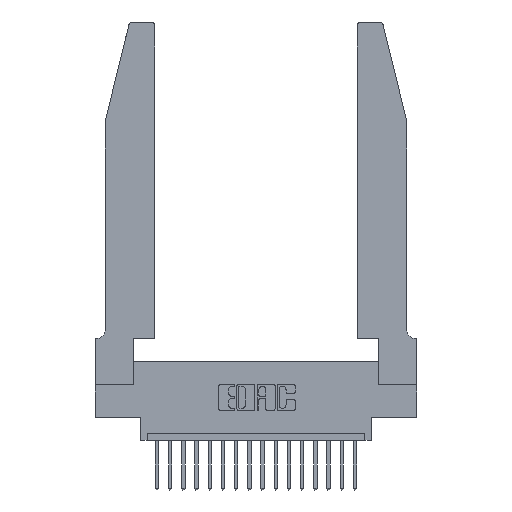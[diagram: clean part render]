
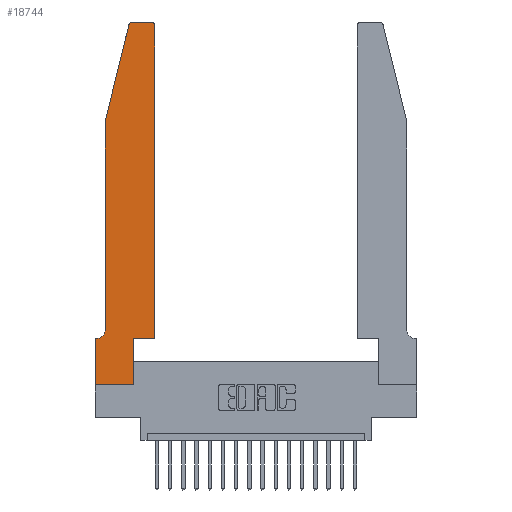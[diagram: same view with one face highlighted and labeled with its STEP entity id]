
A CAD part, top view. The second image highlights one B-rep face of the part: STEP entity #18744.
In plain terms, the highlighted planar face has unit normal (0, 0, 1).
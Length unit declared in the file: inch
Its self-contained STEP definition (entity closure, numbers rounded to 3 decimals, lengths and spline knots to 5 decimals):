
#223 = LINE ( 'NONE', #2592, #8878 ) ;
#569 = ORIENTED_EDGE ( 'NONE', *, *, #1239, .T. ) ;
#579 = CARTESIAN_POINT ( 'NONE',  ( 0., 0., 0.37 ) ) ;
#688 = DIRECTION ( 'NONE',  ( -1., 0., 0. ) ) ;
#765 = LINE ( 'NONE', #579, #12304 ) ;
#1239 = EDGE_CURVE ( 'NONE', #16438, #9061, #16453, .T. ) ;
#1571 = FACE_OUTER_BOUND ( 'NONE', #16148, .T. ) ;
#1942 = EDGE_CURVE ( 'NONE', #5717, #12762, #223, .T. ) ;
#2067 = EDGE_CURVE ( 'NONE', #15623, #10496, #10106, .T. ) ;
#2228 = VERTEX_POINT ( 'NONE', #17329 ) ;
#2475 = VERTEX_POINT ( 'NONE', #11932 ) ;
#2592 = CARTESIAN_POINT ( 'NONE',  ( 0.2865, 0.35, 0.37 ) ) ;
#3256 = CIRCLE ( 'NONE', #19021, 0.03 ) ;
#3722 = ORIENTED_EDGE ( 'NONE', *, *, #9551, .T. ) ;
#4194 = EDGE_CURVE ( 'NONE', #2475, #15623, #9070, .T. ) ;
#4351 = VECTOR ( 'NONE', #6254, 39.37008 ) ;
#4526 = ORIENTED_EDGE ( 'NONE', *, *, #7225, .T. ) ;
#4527 = CARTESIAN_POINT ( 'NONE',  ( 0.4505, 0.35, 0.37 ) ) ;
#4788 = VECTOR ( 'NONE', #15530, 39.37008 ) ;
#5041 = LINE ( 'NONE', #4527, #7008 ) ;
#5350 = CARTESIAN_POINT ( 'NONE',  ( 0., 0.35, 0.37 ) ) ;
#5684 = VECTOR ( 'NONE', #13854, 39.37008 ) ;
#5717 = VERTEX_POINT ( 'NONE', #15624 ) ;
#5984 = CARTESIAN_POINT ( 'NONE',  ( 0.4205, 2.75, 0.37 ) ) ;
#6019 = AXIS2_PLACEMENT_3D ( 'NONE', #13675, #12024, #8843 ) ;
#6124 = CIRCLE ( 'NONE', #13104, 0.07 ) ;
#6254 = DIRECTION ( 'NONE',  ( -0.239, -0.971, 0. ) ) ;
#6587 = ORIENTED_EDGE ( 'NONE', *, *, #8538, .T. ) ;
#6617 = CARTESIAN_POINT ( 'NONE',  ( 0.2605, 2.75, 0.37 ) ) ;
#7008 = VECTOR ( 'NONE', #14106, 39.37008 ) ;
#7038 = CARTESIAN_POINT ( 'NONE',  ( 0.0755, 0.35, 0.37 ) ) ;
#7173 = CARTESIAN_POINT ( 'NONE',  ( 0.0755, 2., 0.37 ) ) ;
#7225 = EDGE_CURVE ( 'NONE', #2228, #5717, #9192, .T. ) ;
#7526 = ORIENTED_EDGE ( 'NONE', *, *, #11359, .T. ) ;
#7937 = VECTOR ( 'NONE', #13583, 39.37008 ) ;
#8290 = VECTOR ( 'NONE', #688, 39.37008 ) ;
#8363 = CARTESIAN_POINT ( 'NONE',  ( 0.4505, 2.72, 0.37 ) ) ;
#8538 = EDGE_CURVE ( 'NONE', #9028, #2228, #765, .T. ) ;
#8763 = PLANE ( 'NONE',  #6019 ) ;
#8843 = DIRECTION ( 'NONE',  ( 1., 0., 0. ) ) ;
#8878 = VECTOR ( 'NONE', #14405, 39.37008 ) ;
#8976 = LINE ( 'NONE', #9428, #4788 ) ;
#9028 = VERTEX_POINT ( 'NONE', #5350 ) ;
#9061 = VERTEX_POINT ( 'NONE', #5984 ) ;
#9070 = LINE ( 'NONE', #9418, #4351 ) ;
#9118 = CARTESIAN_POINT ( 'NONE',  ( 0.2865, 0.35, 0.37 ) ) ;
#9192 = LINE ( 'NONE', #12067, #7937 ) ;
#9417 = DIRECTION ( 'NONE',  ( 0., 0., 1. ) ) ;
#9418 = CARTESIAN_POINT ( 'NONE',  ( 0.0755, 2., 0.37 ) ) ;
#9428 = CARTESIAN_POINT ( 'NONE',  ( 0.4505, 0.35, 0.37 ) ) ;
#9455 = EDGE_CURVE ( 'NONE', #13883, #9028, #14719, .T. ) ;
#9549 = CARTESIAN_POINT ( 'NONE',  ( 0.4205, 2.72, 0.37 ) ) ;
#9551 = EDGE_CURVE ( 'NONE', #9061, #19842, #10019, .T. ) ;
#9976 = CARTESIAN_POINT ( 'NONE',  ( 0.0055, 0.35, 0.37 ) ) ;
#10019 = LINE ( 'NONE', #6617, #8290 ) ;
#10106 = LINE ( 'NONE', #12341, #5684 ) ;
#10487 = ORIENTED_EDGE ( 'NONE', *, *, #1942, .T. ) ;
#10496 = VERTEX_POINT ( 'NONE', #10815 ) ;
#10815 = CARTESIAN_POINT ( 'NONE',  ( 0.0755, 0.42, 0.37 ) ) ;
#11260 = EDGE_CURVE ( 'NONE', #12642, #16438, #5041, .T. ) ;
#11359 = EDGE_CURVE ( 'NONE', #19842, #2475, #3256, .T. ) ;
#11646 = ORIENTED_EDGE ( 'NONE', *, *, #11260, .T. ) ;
#11932 = CARTESIAN_POINT ( 'NONE',  ( 0.25487, 2.72718, 0.37 ) ) ;
#11948 = CARTESIAN_POINT ( 'NONE',  ( 0.4505, 0.35, 0.37 ) ) ;
#12024 = DIRECTION ( 'NONE',  ( 0., 0., 1. ) ) ;
#12067 = CARTESIAN_POINT ( 'NONE',  ( 0., 0., 0.37 ) ) ;
#12109 = ORIENTED_EDGE ( 'NONE', *, *, #2067, .T. ) ;
#12141 = ORIENTED_EDGE ( 'NONE', *, *, #14295, .T. ) ;
#12245 = ORIENTED_EDGE ( 'NONE', *, *, #19434, .T. ) ;
#12304 = VECTOR ( 'NONE', #19263, 39.37008 ) ;
#12341 = CARTESIAN_POINT ( 'NONE',  ( 0.0755, 2., 0.37 ) ) ;
#12447 = DIRECTION ( 'NONE',  ( 1., 0., 0. ) ) ;
#12642 = VERTEX_POINT ( 'NONE', #11948 ) ;
#12649 = DIRECTION ( 'NONE',  ( 0., 0., 1. ) ) ;
#12762 = VERTEX_POINT ( 'NONE', #9118 ) ;
#13104 = AXIS2_PLACEMENT_3D ( 'NONE', #14772, #19513, #16444 ) ;
#13583 = DIRECTION ( 'NONE',  ( 1., 0., 0. ) ) ;
#13675 = CARTESIAN_POINT ( 'NONE',  ( 0., 0.35, 0.37 ) ) ;
#13854 = DIRECTION ( 'NONE',  ( 0., -1., 0. ) ) ;
#13883 = VERTEX_POINT ( 'NONE', #9976 ) ;
#14106 = DIRECTION ( 'NONE',  ( 0., 1., 0. ) ) ;
#14295 = EDGE_CURVE ( 'NONE', #10496, #13883, #6124, .T. ) ;
#14405 = DIRECTION ( 'NONE',  ( 0., 1., 0. ) ) ;
#14719 = LINE ( 'NONE', #7038, #17928 ) ;
#14772 = CARTESIAN_POINT ( 'NONE',  ( 0.0055, 0.42, 0.37 ) ) ;
#15159 = ORIENTED_EDGE ( 'NONE', *, *, #4194, .T. ) ;
#15530 = DIRECTION ( 'NONE',  ( 1., 0., 0. ) ) ;
#15623 = VERTEX_POINT ( 'NONE', #7173 ) ;
#15624 = CARTESIAN_POINT ( 'NONE',  ( 0.2865, 0., 0.37 ) ) ;
#15784 = CARTESIAN_POINT ( 'NONE',  ( 0.284, 2.72, 0.37 ) ) ;
#16148 = EDGE_LOOP ( 'NONE', ( #3722, #7526, #15159, #12109, #12141, #16815, #6587, #4526, #10487, #12245, #11646, #569 ) ) ;
#16438 = VERTEX_POINT ( 'NONE', #8363 ) ;
#16444 = DIRECTION ( 'NONE',  ( -1., 0., 0. ) ) ;
#16453 = CIRCLE ( 'NONE', #17976, 0.03 ) ;
#16577 = DIRECTION ( 'NONE',  ( -1., 0., 0. ) ) ;
#16815 = ORIENTED_EDGE ( 'NONE', *, *, #9455, .T. ) ;
#17329 = CARTESIAN_POINT ( 'NONE',  ( 0., 0., 0.37 ) ) ;
#17356 = DIRECTION ( 'NONE',  ( 1., 0., 0. ) ) ;
#17928 = VECTOR ( 'NONE', #16577, 39.37008 ) ;
#17976 = AXIS2_PLACEMENT_3D ( 'NONE', #9549, #9417, #12447 ) ;
#18744 = ADVANCED_FACE ( 'NONE', ( #1571 ), #8763, .T. ) ;
#19021 = AXIS2_PLACEMENT_3D ( 'NONE', #15784, #12649, #17356 ) ;
#19263 = DIRECTION ( 'NONE',  ( 0., -1., 0. ) ) ;
#19434 = EDGE_CURVE ( 'NONE', #12762, #12642, #8976, .T. ) ;
#19513 = DIRECTION ( 'NONE',  ( 0., 0., -1. ) ) ;
#19617 = CARTESIAN_POINT ( 'NONE',  ( 0.284, 2.75, 0.37 ) ) ;
#19842 = VERTEX_POINT ( 'NONE', #19617 ) ;
